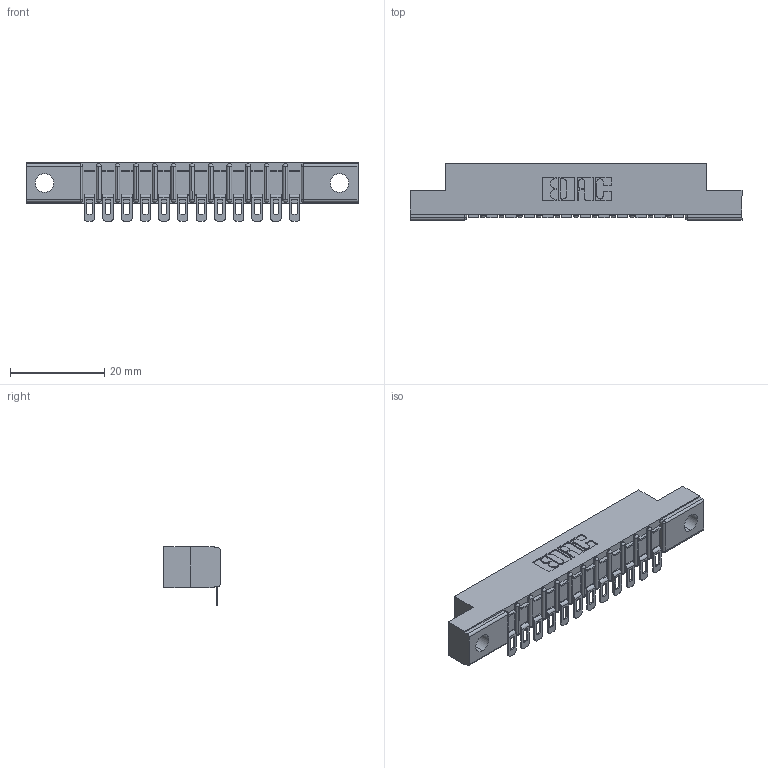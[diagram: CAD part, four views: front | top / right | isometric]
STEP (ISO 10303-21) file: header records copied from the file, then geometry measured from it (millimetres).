
FILE_DESCRIPTION (( 'STEP AP203' ), '1' );
FILE_NAME ('357-012-454-104.STEP', '2020-09-30T12:36:43', ( '' ), ( '' ), 'SwSTEP 2.0', 'SolidWorks 2020', '' );
FILE_SCHEMA (( 'CONFIG_CONTROL_DESIGN' ));
Length unit declared in the file: inch
Products named in the file (3): 307 Part_.156 Dia Mounting Holes; 357-012-454-104; 307-290-002_554
Assembly tree (13 placements, depth 2):
  357-012-454-104
    307 Part_.156 Dia Mounting Holes
    307-290-002_554  x12
Bounding box: 70.56 x 12.01 x 12.52 mm (x, y, z)
Volume: 4551.5 mm3; surface area: 7662.4 mm2
Topology: 13 solids, 13 shells, 1117 faces, 3395 edges, 2226 vertices
Faces by surface type: plane 636, cylinder 455, sphere 26
Entity records: 15369 total; most frequent: CARTESIAN_POINT 2592, ORIENTED_EDGE 2580, DIRECTION 2530, EDGE_CURVE 1290, LINE 974, VECTOR 974, VERTEX_POINT 840, AXIS2_PLACEMENT_3D 778
